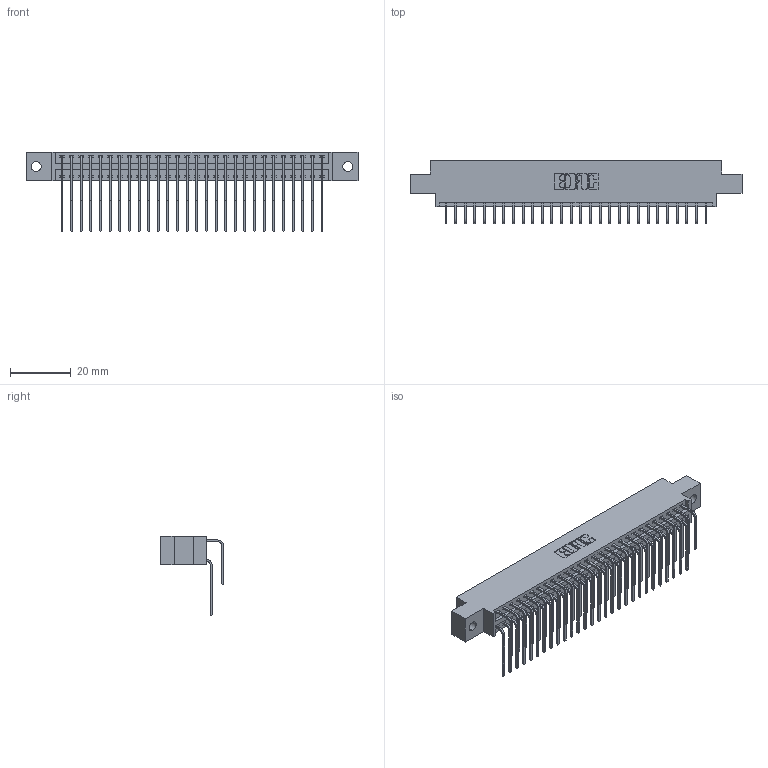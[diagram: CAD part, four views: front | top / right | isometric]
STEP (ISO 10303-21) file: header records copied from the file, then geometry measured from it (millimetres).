
FILE_DESCRIPTION (( 'STEP AP203' ), '1' );
FILE_NAME ('396-056-559-802.STEP', '2018-09-08T10:31:55', ( '' ), ( '' ), 'SwSTEP 2.0', 'SolidWorks 2016', '' );
FILE_SCHEMA (( 'CONFIG_CONTROL_DESIGN' ));
Length unit declared in the file: inch
Products named in the file (4): 346 Part_0.170 Offset - 0.128 Dia; 345-292-001_558 559 Tail - 1; 345-292-001_559 Tail - 2; 396-056-559-802
Assembly tree (57 placements, depth 2):
  396-056-559-802
    346 Part_0.170 Offset - 0.128 Dia
    345-292-001_558 559 Tail - 1  x28
    345-292-001_559 Tail - 2  x28
Bounding box: 109.47 x 20.89 x 26.16 mm (x, y, z)
Volume: 10698.1 mm3; surface area: 15945.4 mm2
Topology: 57 solids, 57 shells, 3150 faces, 9357 edges, 6162 vertices
Faces by surface type: plane 2152, cylinder 998
Entity records: 22077 total; most frequent: CARTESIAN_POINT 3711, ORIENTED_EDGE 3594, DIRECTION 3293, EDGE_CURVE 1797, VECTOR 1513, LINE 1513, VERTEX_POINT 1194, AXIS2_PLACEMENT_3D 890
